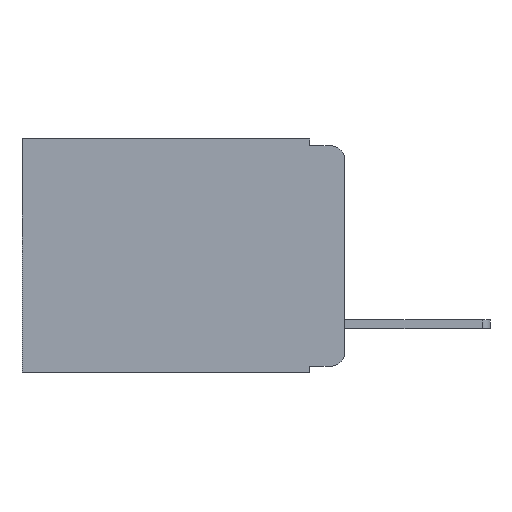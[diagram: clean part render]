
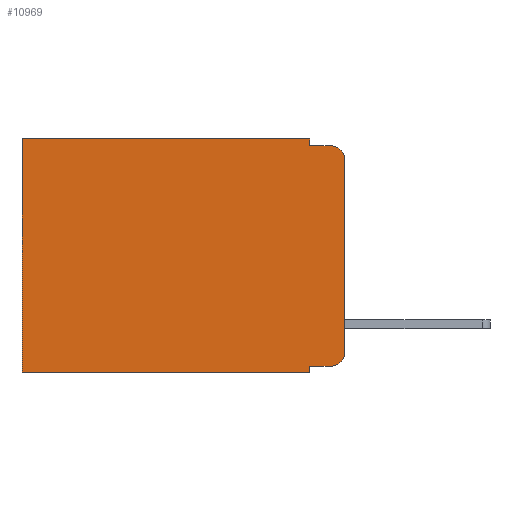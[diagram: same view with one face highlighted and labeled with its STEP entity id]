
A CAD part, left-side view. The second image highlights one B-rep face of the part: STEP entity #10969.
In plain terms, the highlighted planar face has unit normal (-1, 0, 0).
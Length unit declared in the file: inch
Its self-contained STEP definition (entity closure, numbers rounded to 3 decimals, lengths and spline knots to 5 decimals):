
#178 = CARTESIAN_POINT ( 'NONE',  ( 0.298, 0.02, -0.03 ) ) ;
#220 = VERTEX_POINT ( 'NONE', #6547 ) ;
#482 = DIRECTION ( 'NONE',  ( 1., 0., 0. ) ) ;
#499 = EDGE_CURVE ( 'NONE', #12724, #3013, #10601, .T. ) ;
#601 = VERTEX_POINT ( 'NONE', #10936 ) ;
#755 = LINE ( 'NONE', #13755, #6440 ) ;
#946 = ORIENTED_EDGE ( 'NONE', *, *, #12211, .F. ) ;
#1505 = DIRECTION ( 'NONE',  ( 0., 0., -1. ) ) ;
#1586 = EDGE_CURVE ( 'NONE', #9932, #601, #5515, .T. ) ;
#1642 = CARTESIAN_POINT ( 'NONE',  ( 0.298, 0., -0.313 ) ) ;
#1851 = EDGE_CURVE ( 'NONE', #220, #11759, #13969, .T. ) ;
#1950 = CARTESIAN_POINT ( 'NONE',  ( 0.298, 0.02, -0.01 ) ) ;
#2088 = CARTESIAN_POINT ( 'NONE',  ( 0.298, 0.02, -0.313 ) ) ;
#2221 = VERTEX_POINT ( 'NONE', #6489 ) ;
#2684 = VERTEX_POINT ( 'NONE', #11896 ) ;
#2804 = DIRECTION ( 'NONE',  ( -1., 0., 0. ) ) ;
#2874 = AXIS2_PLACEMENT_3D ( 'NONE', #2088, #9953, #3270 ) ;
#2954 = EDGE_CURVE ( 'NONE', #2684, #11139, #12029, .T. ) ;
#3013 = VERTEX_POINT ( 'NONE', #1950 ) ;
#3067 = CARTESIAN_POINT ( 'NONE',  ( 0.298, 0., 0. ) ) ;
#3270 = DIRECTION ( 'NONE',  ( 0., 0., -1. ) ) ;
#3295 = CARTESIAN_POINT ( 'NONE',  ( 0.298, 0.02, -0.333 ) ) ;
#3708 = ORIENTED_EDGE ( 'NONE', *, *, #1586, .F. ) ;
#4258 = DIRECTION ( 'NONE',  ( 0., 1., 0. ) ) ;
#4512 = FACE_OUTER_BOUND ( 'NONE', #5396, .T. ) ;
#4866 = VERTEX_POINT ( 'NONE', #1642 ) ;
#5396 = EDGE_LOOP ( 'NONE', ( #946, #8681, #11421, #3708, #8915, #6972, #5591, #12369, #9373, #12512 ) ) ;
#5515 = LINE ( 'NONE', #13013, #8132 ) ;
#5571 = EDGE_CURVE ( 'NONE', #2684, #2221, #755, .T. ) ;
#5591 = ORIENTED_EDGE ( 'NONE', *, *, #10449, .F. ) ;
#6137 = PLANE ( 'NONE',  #11374 ) ;
#6295 = VECTOR ( 'NONE', #4258, 39.37008 ) ;
#6331 = DIRECTION ( 'NONE',  ( 0., -1., 0. ) ) ;
#6440 = VECTOR ( 'NONE', #8476, 39.37008 ) ;
#6489 = CARTESIAN_POINT ( 'NONE',  ( 0.298, 0.051, -0.343 ) ) ;
#6547 = CARTESIAN_POINT ( 'NONE',  ( 0.298, 0.473, 0. ) ) ;
#6694 = CARTESIAN_POINT ( 'NONE',  ( 0.298, 0.473, -0.343 ) ) ;
#6972 = ORIENTED_EDGE ( 'NONE', *, *, #1851, .T. ) ;
#6987 = DIRECTION ( 'NONE',  ( 0., 0., -1. ) ) ;
#7266 = CARTESIAN_POINT ( 'NONE',  ( 0.298, 0., 0. ) ) ;
#7371 = DIRECTION ( 'NONE',  ( 0., 0., -1. ) ) ;
#7443 = DIRECTION ( 'NONE',  ( 0., 1., 0. ) ) ;
#7838 = VECTOR ( 'NONE', #7443, 39.37008 ) ;
#8132 = VECTOR ( 'NONE', #1505, 39.37008 ) ;
#8179 = LINE ( 'NONE', #12849, #7838 ) ;
#8373 = DIRECTION ( 'NONE',  ( 0., 0., -1. ) ) ;
#8476 = DIRECTION ( 'NONE',  ( 0., 0., -1. ) ) ;
#8657 = CARTESIAN_POINT ( 'NONE',  ( 0.298, 0.051, 0. ) ) ;
#8681 = ORIENTED_EDGE ( 'NONE', *, *, #499, .T. ) ;
#8839 = EDGE_CURVE ( 'NONE', #11139, #4866, #12166, .T. ) ;
#8915 = ORIENTED_EDGE ( 'NONE', *, *, #12828, .T. ) ;
#8986 = AXIS2_PLACEMENT_3D ( 'NONE', #178, #2804, #6987 ) ;
#9145 = VECTOR ( 'NONE', #6331, 39.37008 ) ;
#9373 = ORIENTED_EDGE ( 'NONE', *, *, #2954, .T. ) ;
#9647 = CARTESIAN_POINT ( 'NONE',  ( 0.298, 0., -0.03 ) ) ;
#9932 = VERTEX_POINT ( 'NONE', #8657 ) ;
#9953 = DIRECTION ( 'NONE',  ( -1., 0., 0. ) ) ;
#10449 = EDGE_CURVE ( 'NONE', #2221, #11759, #8179, .T. ) ;
#10581 = LINE ( 'NONE', #3067, #13349 ) ;
#10601 = CIRCLE ( 'NONE', #8986, 0.02 ) ;
#10758 = VECTOR ( 'NONE', #13580, 39.37008 ) ;
#10898 = VECTOR ( 'NONE', #7371, 39.37008 ) ;
#10936 = CARTESIAN_POINT ( 'NONE',  ( 0.298, 0.051, -0.01 ) ) ;
#10969 = ADVANCED_FACE ( 'NONE', ( #4512 ), #6137, .F. ) ;
#11139 = VERTEX_POINT ( 'NONE', #3295 ) ;
#11374 = AXIS2_PLACEMENT_3D ( 'NONE', #7266, #482, #8373 ) ;
#11421 = ORIENTED_EDGE ( 'NONE', *, *, #11986, .F. ) ;
#11759 = VERTEX_POINT ( 'NONE', #6694 ) ;
#11896 = CARTESIAN_POINT ( 'NONE',  ( 0.298, 0.051, -0.333 ) ) ;
#11952 = CARTESIAN_POINT ( 'NONE',  ( 0.298, 0., 0. ) ) ;
#11986 = EDGE_CURVE ( 'NONE', #601, #3013, #13839, .T. ) ;
#12029 = LINE ( 'NONE', #13740, #9145 ) ;
#12141 = LINE ( 'NONE', #11952, #6295 ) ;
#12166 = CIRCLE ( 'NONE', #2874, 0.02 ) ;
#12211 = EDGE_CURVE ( 'NONE', #12724, #4866, #10581, .T. ) ;
#12369 = ORIENTED_EDGE ( 'NONE', *, *, #5571, .F. ) ;
#12512 = ORIENTED_EDGE ( 'NONE', *, *, #8839, .T. ) ;
#12577 = CARTESIAN_POINT ( 'NONE',  ( 0.298, 0.051, -0.01 ) ) ;
#12724 = VERTEX_POINT ( 'NONE', #9647 ) ;
#12828 = EDGE_CURVE ( 'NONE', #9932, #220, #12141, .T. ) ;
#12849 = CARTESIAN_POINT ( 'NONE',  ( 0.298, 0., -0.343 ) ) ;
#13013 = CARTESIAN_POINT ( 'NONE',  ( 0.298, 0.051, 0. ) ) ;
#13349 = VECTOR ( 'NONE', #13975, 39.37008 ) ;
#13580 = DIRECTION ( 'NONE',  ( 0., -1., 0. ) ) ;
#13740 = CARTESIAN_POINT ( 'NONE',  ( 0.298, 0.051, -0.333 ) ) ;
#13744 = CARTESIAN_POINT ( 'NONE',  ( 0.298, 0.473, 0. ) ) ;
#13755 = CARTESIAN_POINT ( 'NONE',  ( 0.298, 0.051, 0. ) ) ;
#13839 = LINE ( 'NONE', #12577, #10758 ) ;
#13969 = LINE ( 'NONE', #13744, #10898 ) ;
#13975 = DIRECTION ( 'NONE',  ( 0., 0., -1. ) ) ;
